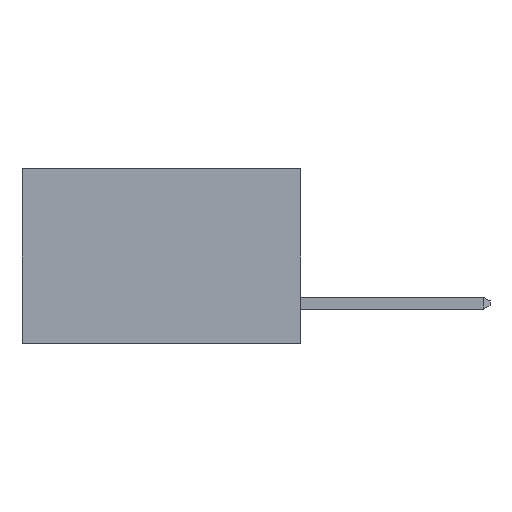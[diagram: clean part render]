
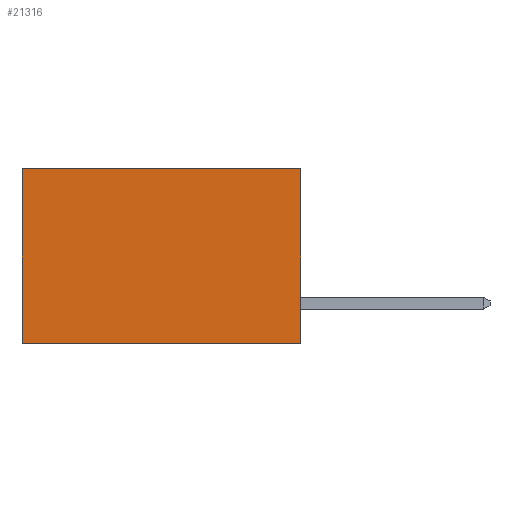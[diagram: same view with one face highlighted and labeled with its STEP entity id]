
A CAD part, left-side view. The second image highlights one B-rep face of the part: STEP entity #21316.
In plain terms, the highlighted planar face has unit normal (-1, 0, 0).
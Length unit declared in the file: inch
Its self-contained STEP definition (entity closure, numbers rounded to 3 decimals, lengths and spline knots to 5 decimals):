
#1191 = EDGE_CURVE ( 'NONE', #15357, #12727, #15742, .T. ) ;
#2135 = DIRECTION ( 'NONE',  ( 0., 0., -1. ) ) ;
#2614 = FACE_OUTER_BOUND ( 'NONE', #4662, .T. ) ;
#3029 = CARTESIAN_POINT ( 'NONE',  ( 0.277, 0., 0. ) ) ;
#3957 = EDGE_CURVE ( 'NONE', #15357, #6036, #17159, .T. ) ;
#4531 = CARTESIAN_POINT ( 'NONE',  ( 0.277, 0., -0.37 ) ) ;
#4612 = CARTESIAN_POINT ( 'NONE',  ( 0.277, 0., -0.37 ) ) ;
#4662 = EDGE_LOOP ( 'NONE', ( #19322, #12902, #16693, #8546 ) ) ;
#5452 = PLANE ( 'NONE',  #11373 ) ;
#6036 = VERTEX_POINT ( 'NONE', #4531 ) ;
#6707 = EDGE_CURVE ( 'NONE', #6036, #10568, #22211, .T. ) ;
#7704 = DIRECTION ( 'NONE',  ( 0., 1., 0. ) ) ;
#8546 = ORIENTED_EDGE ( 'NONE', *, *, #1191, .T. ) ;
#8979 = CARTESIAN_POINT ( 'NONE',  ( 0.277, 0., 0. ) ) ;
#9423 = DIRECTION ( 'NONE',  ( 0., 0., -1. ) ) ;
#9769 = LINE ( 'NONE', #19952, #14395 ) ;
#10324 = CARTESIAN_POINT ( 'NONE',  ( 0.277, 0.59, 0. ) ) ;
#10568 = VERTEX_POINT ( 'NONE', #16566 ) ;
#11293 = VECTOR ( 'NONE', #24685, 39.37008 ) ;
#11373 = AXIS2_PLACEMENT_3D ( 'NONE', #15288, #21298, #9423 ) ;
#12727 = VERTEX_POINT ( 'NONE', #10324 ) ;
#12902 = ORIENTED_EDGE ( 'NONE', *, *, #6707, .F. ) ;
#14395 = VECTOR ( 'NONE', #2135, 39.37008 ) ;
#15288 = CARTESIAN_POINT ( 'NONE',  ( 0.277, 0., -0.37 ) ) ;
#15357 = VERTEX_POINT ( 'NONE', #8979 ) ;
#15698 = EDGE_CURVE ( 'NONE', #12727, #10568, #9769, .T. ) ;
#15742 = LINE ( 'NONE', #3029, #20386 ) ;
#16483 = DIRECTION ( 'NONE',  ( 0., 1., 0. ) ) ;
#16566 = CARTESIAN_POINT ( 'NONE',  ( 0.277, 0.59, -0.37 ) ) ;
#16693 = ORIENTED_EDGE ( 'NONE', *, *, #3957, .F. ) ;
#17159 = LINE ( 'NONE', #24894, #11293 ) ;
#19322 = ORIENTED_EDGE ( 'NONE', *, *, #15698, .T. ) ;
#19952 = CARTESIAN_POINT ( 'NONE',  ( 0.277, 0.59, -0.37 ) ) ;
#20386 = VECTOR ( 'NONE', #7704, 39.37008 ) ;
#21298 = DIRECTION ( 'NONE',  ( 1., 0., 0. ) ) ;
#21316 = ADVANCED_FACE ( 'NONE', ( #2614 ), #5452, .F. ) ;
#21580 = VECTOR ( 'NONE', #16483, 39.37008 ) ;
#22211 = LINE ( 'NONE', #4612, #21580 ) ;
#24685 = DIRECTION ( 'NONE',  ( 0., 0., -1. ) ) ;
#24894 = CARTESIAN_POINT ( 'NONE',  ( 0.277, 0., -0.37 ) ) ;
